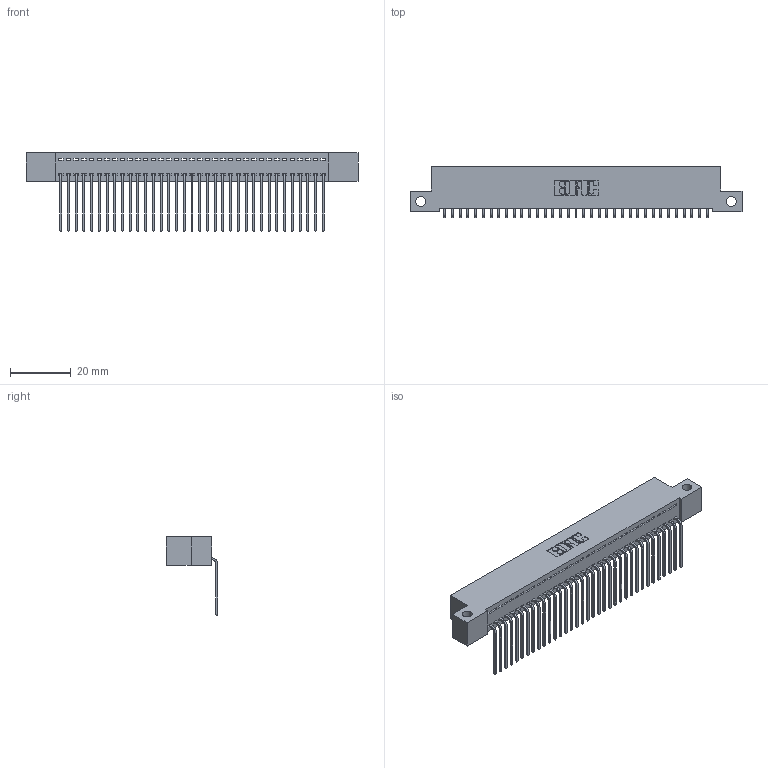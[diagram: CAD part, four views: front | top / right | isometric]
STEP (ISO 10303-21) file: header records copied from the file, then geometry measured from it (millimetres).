
FILE_DESCRIPTION (( 'STEP AP203' ), '1' );
FILE_NAME ('342-035-559-112.STEP', '2019-10-02T13:01:57', ( '' ), ( '' ), 'SwSTEP 2.0', 'SolidWorks 2016', '' );
FILE_SCHEMA (( 'CONFIG_CONTROL_DESIGN' ));
Length unit declared in the file: inch
Products named in the file (3): 342-035-559-112; 342 Part_Side Mount; 345-292-001_558 559 Tail - 1
Assembly tree (36 placements, depth 2):
  342-035-559-112
    342 Part_Side Mount
    345-292-001_558 559 Tail - 1  x35
Bounding box: 109.22 x 16.83 x 25.78 mm (x, y, z)
Volume: 9593.3 mm3; surface area: 14455.8 mm2
Topology: 36 solids, 36 shells, 2210 faces, 6669 edges, 4398 vertices
Faces by surface type: plane 1606, cylinder 604
Entity records: 22257 total; most frequent: CARTESIAN_POINT 3847, ORIENTED_EDGE 3818, DIRECTION 3259, EDGE_CURVE 1909, LINE 1781, VECTOR 1781, VERTEX_POINT 1270, AXIS2_PLACEMENT_3D 739
